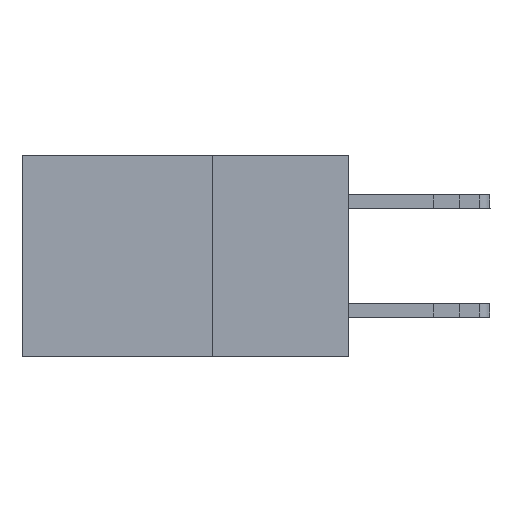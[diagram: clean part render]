
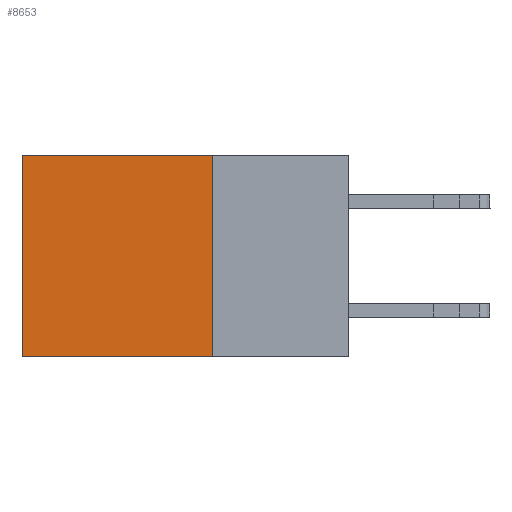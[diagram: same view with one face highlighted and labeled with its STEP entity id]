
A CAD part, left-side view. The second image highlights one B-rep face of the part: STEP entity #8653.
In plain terms, the highlighted planar face has unit normal (-1, 0, 0).
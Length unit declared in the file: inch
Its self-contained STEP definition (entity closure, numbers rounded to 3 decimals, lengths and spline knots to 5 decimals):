
#1314 = DIRECTION ( 'NONE',  ( 0., 1., 0. ) ) ;
#1451 = CARTESIAN_POINT ( 'NONE',  ( 0.2615, 0.6, -0.37 ) ) ;
#1505 = CARTESIAN_POINT ( 'NONE',  ( 0.2615, 0.25, -0.37 ) ) ;
#2004 = VERTEX_POINT ( 'NONE', #11117 ) ;
#2079 = EDGE_CURVE ( 'NONE', #2004, #4021, #4017, .T. ) ;
#2273 = EDGE_CURVE ( 'NONE', #2004, #10549, #10612, .T. ) ;
#2305 = LINE ( 'NONE', #9008, #2946 ) ;
#2306 = EDGE_CURVE ( 'NONE', #10549, #3380, #9810, .T. ) ;
#2461 = FACE_OUTER_BOUND ( 'NONE', #8590, .T. ) ;
#2946 = VECTOR ( 'NONE', #10742, 39.37008 ) ;
#3380 = VERTEX_POINT ( 'NONE', #4581 ) ;
#3494 = EDGE_CURVE ( 'NONE', #4021, #3380, #2305, .T. ) ;
#4017 = LINE ( 'NONE', #9438, #11488 ) ;
#4021 = VERTEX_POINT ( 'NONE', #1505 ) ;
#4328 = CARTESIAN_POINT ( 'NONE',  ( 0.2615, 0.6, 0. ) ) ;
#4401 = CARTESIAN_POINT ( 'NONE',  ( 0.2615, 0.25, -0.37 ) ) ;
#4581 = CARTESIAN_POINT ( 'NONE',  ( 0.2615, 0.6, -0.37 ) ) ;
#4965 = ORIENTED_EDGE ( 'NONE', *, *, #3494, .F. ) ;
#5065 = VECTOR ( 'NONE', #8900, 39.37008 ) ;
#5230 = AXIS2_PLACEMENT_3D ( 'NONE', #4401, #5510, #11850 ) ;
#5510 = DIRECTION ( 'NONE',  ( 1., 0., 0. ) ) ;
#5895 = ORIENTED_EDGE ( 'NONE', *, *, #2306, .T. ) ;
#6373 = PLANE ( 'NONE',  #5230 ) ;
#6837 = DIRECTION ( 'NONE',  ( 0., 0., -1. ) ) ;
#8590 = EDGE_LOOP ( 'NONE', ( #5895, #4965, #9793, #11658 ) ) ;
#8653 = ADVANCED_FACE ( 'NONE', ( #2461 ), #6373, .F. ) ;
#8845 = CARTESIAN_POINT ( 'NONE',  ( 0.2615, 0.25, 0. ) ) ;
#8900 = DIRECTION ( 'NONE',  ( 0., 0., -1. ) ) ;
#8969 = VECTOR ( 'NONE', #1314, 39.37008 ) ;
#9008 = CARTESIAN_POINT ( 'NONE',  ( 0.2615, 0.25, -0.37 ) ) ;
#9438 = CARTESIAN_POINT ( 'NONE',  ( 0.2615, 0.25, -0.37 ) ) ;
#9793 = ORIENTED_EDGE ( 'NONE', *, *, #2079, .F. ) ;
#9810 = LINE ( 'NONE', #1451, #5065 ) ;
#10549 = VERTEX_POINT ( 'NONE', #4328 ) ;
#10612 = LINE ( 'NONE', #8845, #8969 ) ;
#10742 = DIRECTION ( 'NONE',  ( 0., 1., 0. ) ) ;
#11117 = CARTESIAN_POINT ( 'NONE',  ( 0.2615, 0.25, 0. ) ) ;
#11488 = VECTOR ( 'NONE', #6837, 39.37008 ) ;
#11658 = ORIENTED_EDGE ( 'NONE', *, *, #2273, .T. ) ;
#11850 = DIRECTION ( 'NONE',  ( 0., 0., -1. ) ) ;
